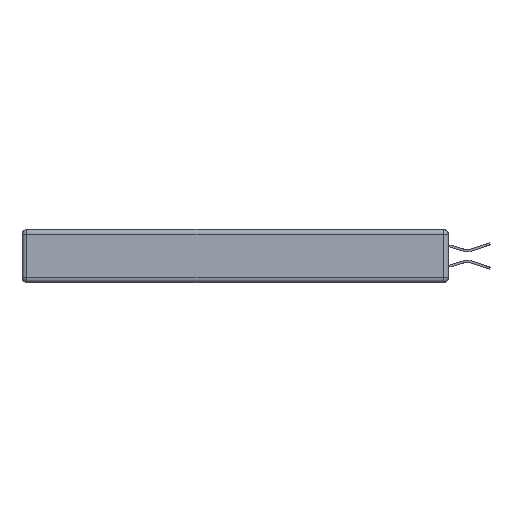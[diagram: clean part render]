
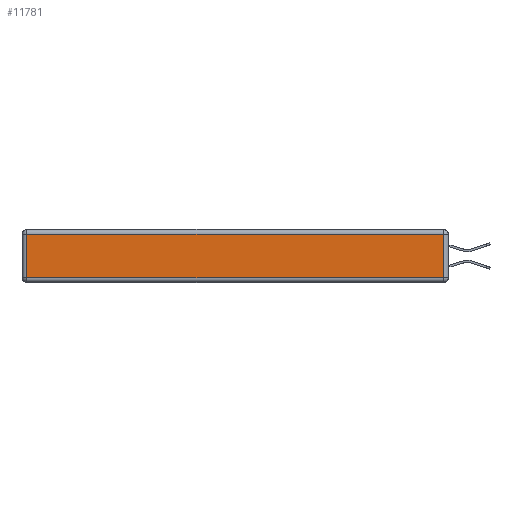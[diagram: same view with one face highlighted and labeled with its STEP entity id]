
A CAD part, left-side view. The second image highlights one B-rep face of the part: STEP entity #11781.
In plain terms, the highlighted planar face has unit normal (-1, 0, 0).
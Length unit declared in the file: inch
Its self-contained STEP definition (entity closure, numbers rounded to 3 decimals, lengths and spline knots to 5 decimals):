
#1507 = CARTESIAN_POINT ( 'NONE',  ( 0., 0.03, -0.343 ) ) ;
#2047 = EDGE_CURVE ( 'NONE', #11248, #15492, #16664, .T. ) ;
#2384 = EDGE_LOOP ( 'NONE', ( #15952, #2943, #25721, #27691 ) ) ;
#2752 = CARTESIAN_POINT ( 'NONE',  ( 0., 2.72, -0.03 ) ) ;
#2943 = ORIENTED_EDGE ( 'NONE', *, *, #4566, .T. ) ;
#4566 = EDGE_CURVE ( 'NONE', #27273, #11248, #29022, .T. ) ;
#6507 = CARTESIAN_POINT ( 'NONE',  ( 0., 0., -0.313 ) ) ;
#6795 = VERTEX_POINT ( 'NONE', #25988 ) ;
#7083 = VECTOR ( 'NONE', #9041, 39.37008 ) ;
#8887 = VECTOR ( 'NONE', #9053, 39.37008 ) ;
#9041 = DIRECTION ( 'NONE',  ( 0., -1., 0. ) ) ;
#9053 = DIRECTION ( 'NONE',  ( 0., 0., -1. ) ) ;
#11248 = VERTEX_POINT ( 'NONE', #31019 ) ;
#11781 = ADVANCED_FACE ( 'NONE', ( #13664 ), #25160, .T. ) ;
#13664 = FACE_OUTER_BOUND ( 'NONE', #2384, .T. ) ;
#13910 = VECTOR ( 'NONE', #20333, 39.37008 ) ;
#15202 = DIRECTION ( 'NONE',  ( 0., 0., 1. ) ) ;
#15492 = VERTEX_POINT ( 'NONE', #2752 ) ;
#15952 = ORIENTED_EDGE ( 'NONE', *, *, #26974, .T. ) ;
#16664 = LINE ( 'NONE', #30396, #13910 ) ;
#17828 = DIRECTION ( 'NONE',  ( -1., 0., 0. ) ) ;
#20333 = DIRECTION ( 'NONE',  ( 0., 1., 0. ) ) ;
#20463 = LINE ( 'NONE', #6507, #7083 ) ;
#20605 = EDGE_CURVE ( 'NONE', #15492, #6795, #25772, .T. ) ;
#23118 = CARTESIAN_POINT ( 'NONE',  ( 0., 0.03, -0.313 ) ) ;
#25160 = PLANE ( 'NONE',  #32081 ) ;
#25267 = CARTESIAN_POINT ( 'NONE',  ( 0., 0., -0.343 ) ) ;
#25721 = ORIENTED_EDGE ( 'NONE', *, *, #2047, .T. ) ;
#25772 = LINE ( 'NONE', #26265, #8887 ) ;
#25988 = CARTESIAN_POINT ( 'NONE',  ( 0., 2.72, -0.313 ) ) ;
#26265 = CARTESIAN_POINT ( 'NONE',  ( 0., 2.72, -0.343 ) ) ;
#26746 = DIRECTION ( 'NONE',  ( 0., 0., 1. ) ) ;
#26974 = EDGE_CURVE ( 'NONE', #6795, #27273, #20463, .T. ) ;
#27273 = VERTEX_POINT ( 'NONE', #23118 ) ;
#27691 = ORIENTED_EDGE ( 'NONE', *, *, #20605, .T. ) ;
#29022 = LINE ( 'NONE', #1507, #30203 ) ;
#30203 = VECTOR ( 'NONE', #26746, 39.37008 ) ;
#30396 = CARTESIAN_POINT ( 'NONE',  ( 0., 2.75, -0.03 ) ) ;
#31019 = CARTESIAN_POINT ( 'NONE',  ( 0., 0.03, -0.03 ) ) ;
#32081 = AXIS2_PLACEMENT_3D ( 'NONE', #25267, #17828, #15202 ) ;
